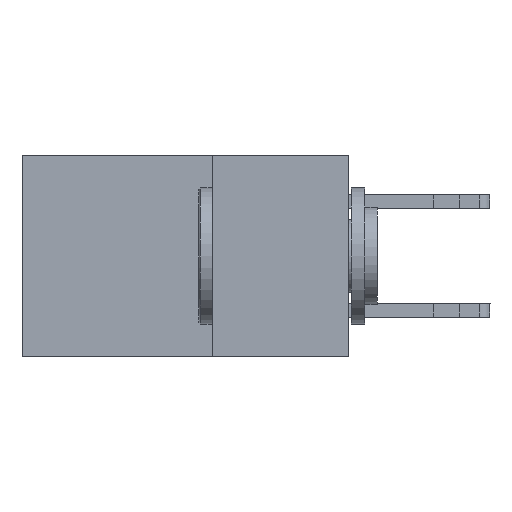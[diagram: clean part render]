
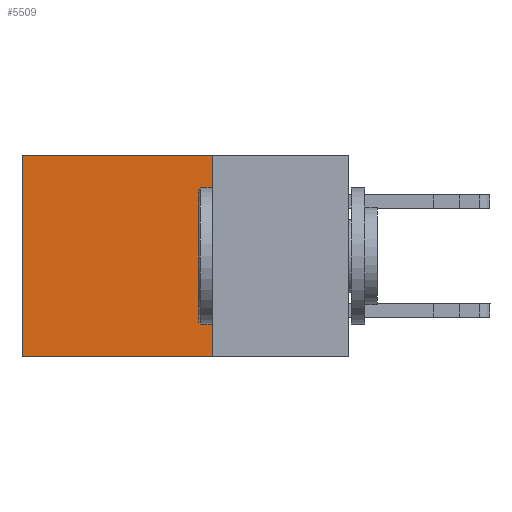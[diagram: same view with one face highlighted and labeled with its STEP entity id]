
A CAD part, left-side view. The second image highlights one B-rep face of the part: STEP entity #5509.
In plain terms, the highlighted planar face has unit normal (-1, 0, 0).
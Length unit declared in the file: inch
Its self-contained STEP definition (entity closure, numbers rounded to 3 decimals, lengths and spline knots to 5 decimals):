
#1071 = LINE ( 'NONE', #5553, #7855 ) ;
#1400 = VERTEX_POINT ( 'NONE', #4667 ) ;
#2764 = VERTEX_POINT ( 'NONE', #11911 ) ;
#2914 = LINE ( 'NONE', #4022, #12562 ) ;
#2998 = LINE ( 'NONE', #12826, #8921 ) ;
#4005 = EDGE_CURVE ( 'NONE', #7070, #8091, #1071, .T. ) ;
#4022 = CARTESIAN_POINT ( 'NONE',  ( 0.2615, 0.6, -0.37 ) ) ;
#4028 = ORIENTED_EDGE ( 'NONE', *, *, #4345, .F. ) ;
#4345 = EDGE_CURVE ( 'NONE', #2764, #1400, #9447, .T. ) ;
#4667 = CARTESIAN_POINT ( 'NONE',  ( 0.2615, 0.6, -0.37 ) ) ;
#5509 = ADVANCED_FACE ( 'NONE', ( #12533 ), #8790, .F. ) ;
#5553 = CARTESIAN_POINT ( 'NONE',  ( 0.2615, 0.25, 0. ) ) ;
#6015 = DIRECTION ( 'NONE',  ( 0., 1., 0. ) ) ;
#6519 = DIRECTION ( 'NONE',  ( 0., 1., 0. ) ) ;
#7070 = VERTEX_POINT ( 'NONE', #8795 ) ;
#7855 = VECTOR ( 'NONE', #6519, 39.37008 ) ;
#7919 = EDGE_LOOP ( 'NONE', ( #14001, #4028, #11919, #9997 ) ) ;
#8091 = VERTEX_POINT ( 'NONE', #15342 ) ;
#8645 = DIRECTION ( 'NONE',  ( 0., 0., -1. ) ) ;
#8651 = DIRECTION ( 'NONE',  ( 1., 0., 0. ) ) ;
#8730 = CARTESIAN_POINT ( 'NONE',  ( 0.2615, 0.25, -0.37 ) ) ;
#8790 = PLANE ( 'NONE',  #9278 ) ;
#8795 = CARTESIAN_POINT ( 'NONE',  ( 0.2615, 0.25, 0. ) ) ;
#8921 = VECTOR ( 'NONE', #10398, 39.37008 ) ;
#9278 = AXIS2_PLACEMENT_3D ( 'NONE', #8730, #8651, #8645 ) ;
#9447 = LINE ( 'NONE', #12388, #15603 ) ;
#9997 = ORIENTED_EDGE ( 'NONE', *, *, #4005, .T. ) ;
#10323 = DIRECTION ( 'NONE',  ( 0., 0., -1. ) ) ;
#10398 = DIRECTION ( 'NONE',  ( 0., 0., -1. ) ) ;
#11911 = CARTESIAN_POINT ( 'NONE',  ( 0.2615, 0.25, -0.37 ) ) ;
#11919 = ORIENTED_EDGE ( 'NONE', *, *, #12716, .F. ) ;
#12388 = CARTESIAN_POINT ( 'NONE',  ( 0.2615, 0.25, -0.37 ) ) ;
#12533 = FACE_OUTER_BOUND ( 'NONE', #7919, .T. ) ;
#12562 = VECTOR ( 'NONE', #10323, 39.37008 ) ;
#12716 = EDGE_CURVE ( 'NONE', #7070, #2764, #2998, .T. ) ;
#12826 = CARTESIAN_POINT ( 'NONE',  ( 0.2615, 0.25, -0.37 ) ) ;
#14001 = ORIENTED_EDGE ( 'NONE', *, *, #15423, .T. ) ;
#15342 = CARTESIAN_POINT ( 'NONE',  ( 0.2615, 0.6, 0. ) ) ;
#15423 = EDGE_CURVE ( 'NONE', #8091, #1400, #2914, .T. ) ;
#15603 = VECTOR ( 'NONE', #6015, 39.37008 ) ;
